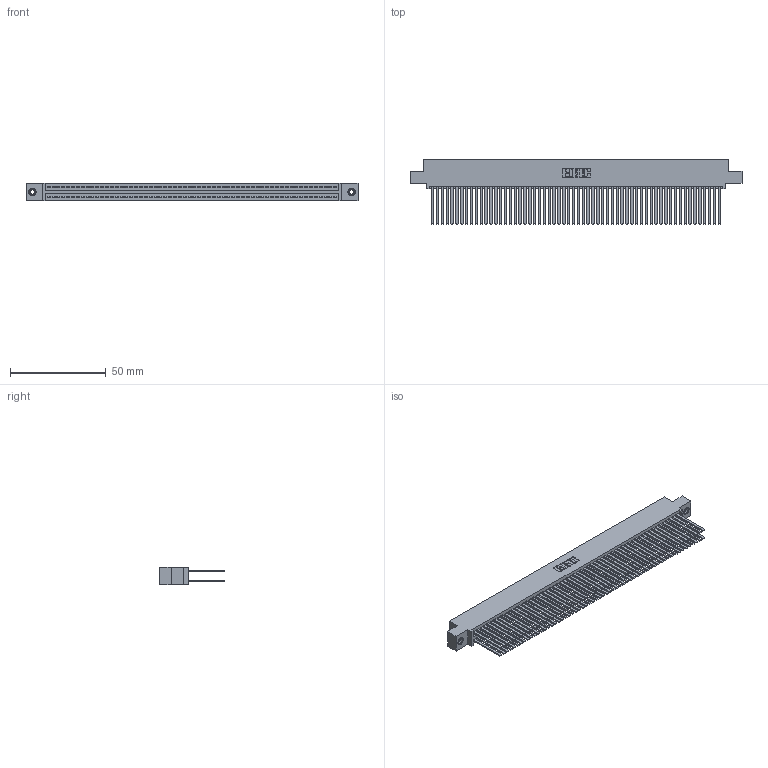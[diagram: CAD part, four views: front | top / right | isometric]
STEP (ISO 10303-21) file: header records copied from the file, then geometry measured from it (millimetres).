
FILE_DESCRIPTION (( 'STEP AP203' ), '1' );
FILE_NAME ('845-120-544-508.STEP', '2018-11-21T04:53:07', ( '' ), ( '' ), 'SwSTEP 2.0', 'SolidWorks 2016', '' );
FILE_SCHEMA (( 'CONFIG_CONTROL_DESIGN' ));
Length unit declared in the file: inch
Products named in the file (4): 845-120-544-508; 845 Part_0.110 Offset - 0.156 Dia-TI; 345-292-001_345-293-144; 345-250-001_345-250-003-102
Assembly tree (123 placements, depth 2):
  845-120-544-508
    845 Part_0.110 Offset - 0.156 Dia-TI
    345-292-001_345-293-144  x120
    345-250-001_345-250-003-102  x2
Bounding box: 173.61 x 33.96 x 9.4 mm (x, y, z)
Volume: 18633.9 mm3; surface area: 32929.3 mm2
Topology: 123 solids, 123 shells, 5470 faces, 16209 edges, 10638 vertices
Faces by surface type: plane 3596, cylinder 1858, cone 12, torus 4
Entity records: 45788 total; most frequent: CARTESIAN_POINT 7639, ORIENTED_EDGE 7566, DIRECTION 6737, EDGE_CURVE 3783, VECTOR 3395, LINE 3395, VERTEX_POINT 2516, AXIS2_PLACEMENT_3D 1671
